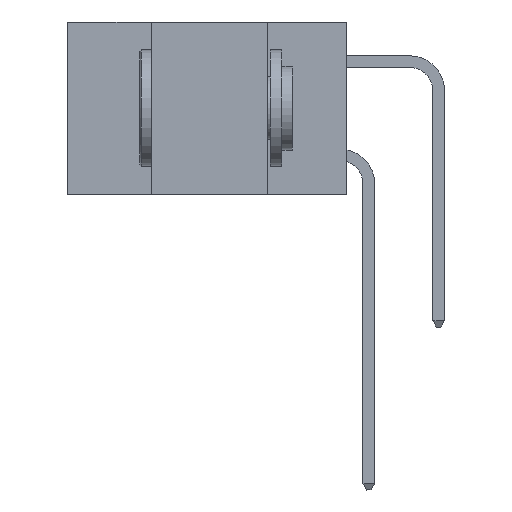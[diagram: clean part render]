
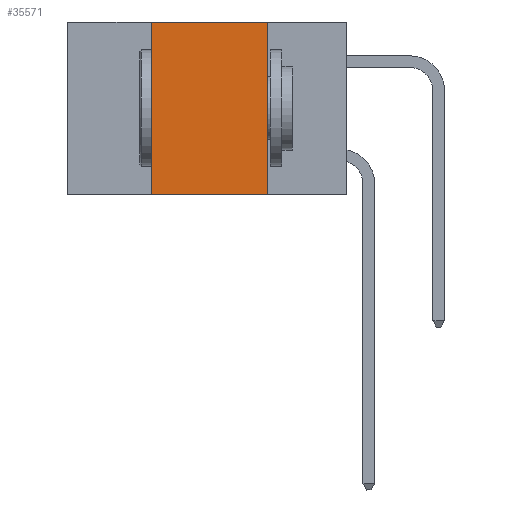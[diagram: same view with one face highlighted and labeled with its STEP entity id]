
A CAD part, left-side view. The second image highlights one B-rep face of the part: STEP entity #35571.
In plain terms, the highlighted planar face has unit normal (-1, 0, 0).
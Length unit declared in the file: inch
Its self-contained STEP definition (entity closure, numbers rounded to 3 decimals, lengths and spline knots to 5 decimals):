
#70 = CARTESIAN_POINT ( 'NONE',  ( 0., 0.17, 0. ) ) ;
#232 = VERTEX_POINT ( 'NONE', #70 ) ;
#1812 = VECTOR ( 'NONE', #14336, 39.37008 ) ;
#2000 = VECTOR ( 'NONE', #36457, 39.37008 ) ;
#2134 = EDGE_LOOP ( 'NONE', ( #35517, #10163, #6210, #5532 ) ) ;
#2540 = VECTOR ( 'NONE', #2635, 39.37008 ) ;
#2635 = DIRECTION ( 'NONE',  ( 0., 0., -1. ) ) ;
#2926 = CARTESIAN_POINT ( 'NONE',  ( 0., 0.42, 0. ) ) ;
#3242 = EDGE_CURVE ( 'NONE', #32940, #232, #19095, .T. ) ;
#5532 = ORIENTED_EDGE ( 'NONE', *, *, #11665, .T. ) ;
#6210 = ORIENTED_EDGE ( 'NONE', *, *, #11136, .F. ) ;
#8157 = EDGE_CURVE ( 'NONE', #232, #12680, #13287, .T. ) ;
#10163 = ORIENTED_EDGE ( 'NONE', *, *, #3242, .F. ) ;
#11136 = EDGE_CURVE ( 'NONE', #28852, #32940, #24371, .T. ) ;
#11665 = EDGE_CURVE ( 'NONE', #28852, #12680, #26574, .T. ) ;
#11991 = AXIS2_PLACEMENT_3D ( 'NONE', #15263, #12360, #21486 ) ;
#12360 = DIRECTION ( 'NONE',  ( 1., 0., 0. ) ) ;
#12680 = VERTEX_POINT ( 'NONE', #31667 ) ;
#13175 = CARTESIAN_POINT ( 'NONE',  ( 0., 0.42, 0. ) ) ;
#13287 = LINE ( 'NONE', #19876, #2540 ) ;
#14336 = DIRECTION ( 'NONE',  ( 0., -1., 0. ) ) ;
#15263 = CARTESIAN_POINT ( 'NONE',  ( 0., 0.6, 0. ) ) ;
#17591 = VECTOR ( 'NONE', #21922, 39.37008 ) ;
#19095 = LINE ( 'NONE', #36077, #2000 ) ;
#19876 = CARTESIAN_POINT ( 'NONE',  ( 0., 0.17, 0. ) ) ;
#21486 = DIRECTION ( 'NONE',  ( 0., 0., -1. ) ) ;
#21922 = DIRECTION ( 'NONE',  ( 0., 0., 1. ) ) ;
#22765 = FACE_OUTER_BOUND ( 'NONE', #2134, .T. ) ;
#24371 = LINE ( 'NONE', #13175, #17591 ) ;
#25577 = CARTESIAN_POINT ( 'NONE',  ( 0., 0.42, -0.37 ) ) ;
#26574 = LINE ( 'NONE', #30520, #1812 ) ;
#28852 = VERTEX_POINT ( 'NONE', #25577 ) ;
#30520 = CARTESIAN_POINT ( 'NONE',  ( 0., 0.6, -0.37 ) ) ;
#31667 = CARTESIAN_POINT ( 'NONE',  ( 0., 0.17, -0.37 ) ) ;
#32584 = PLANE ( 'NONE',  #11991 ) ;
#32940 = VERTEX_POINT ( 'NONE', #2926 ) ;
#35517 = ORIENTED_EDGE ( 'NONE', *, *, #8157, .F. ) ;
#35571 = ADVANCED_FACE ( 'NONE', ( #22765 ), #32584, .F. ) ;
#36077 = CARTESIAN_POINT ( 'NONE',  ( 0., 0.6, 0. ) ) ;
#36457 = DIRECTION ( 'NONE',  ( 0., -1., 0. ) ) ;
